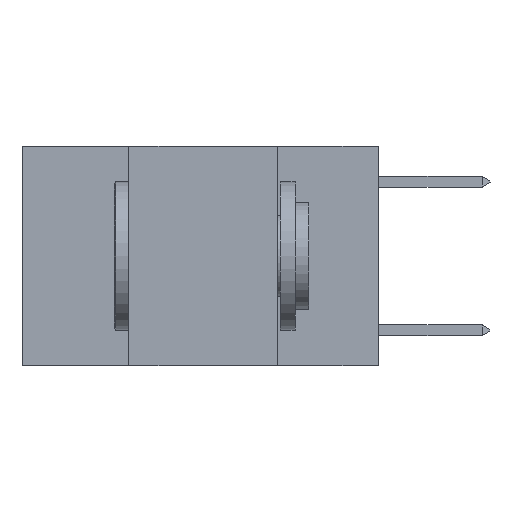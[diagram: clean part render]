
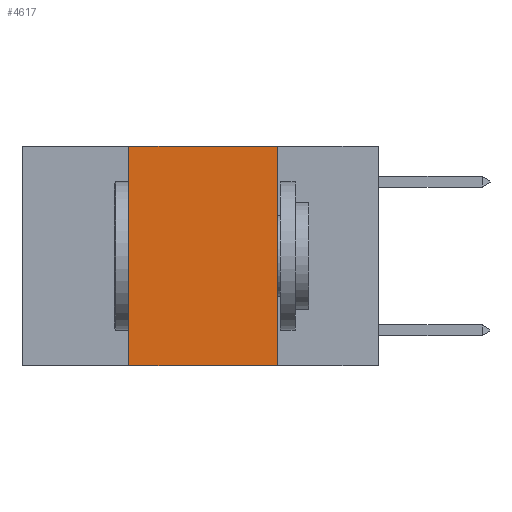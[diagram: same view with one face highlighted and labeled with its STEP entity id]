
A CAD part, left-side view. The second image highlights one B-rep face of the part: STEP entity #4617.
In plain terms, the highlighted planar face has unit normal (-1, 0, 0).
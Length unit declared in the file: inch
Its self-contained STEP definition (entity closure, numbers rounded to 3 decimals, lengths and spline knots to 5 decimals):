
#162 = VERTEX_POINT ( 'NONE', #8802 ) ;
#428 = EDGE_LOOP ( 'NONE', ( #18476, #19750, #6356, #21095 ) ) ;
#827 = VERTEX_POINT ( 'NONE', #20593 ) ;
#1130 = EDGE_CURVE ( 'NONE', #827, #23824, #21213, .T. ) ;
#3015 = DIRECTION ( 'NONE',  ( 0., 0., -1. ) ) ;
#3649 = LINE ( 'NONE', #12258, #13052 ) ;
#3827 = PLANE ( 'NONE',  #18747 ) ;
#4617 = ADVANCED_FACE ( 'NONE', ( #5778 ), #3827, .F. ) ;
#4634 = CARTESIAN_POINT ( 'NONE',  ( 0., 0.42, -0.37 ) ) ;
#5778 = FACE_OUTER_BOUND ( 'NONE', #428, .T. ) ;
#6356 = ORIENTED_EDGE ( 'NONE', *, *, #22737, .F. ) ;
#6431 = VECTOR ( 'NONE', #10769, 39.37008 ) ;
#6537 = DIRECTION ( 'NONE',  ( 0., 0., -1. ) ) ;
#6988 = VECTOR ( 'NONE', #3015, 39.37008 ) ;
#8802 = CARTESIAN_POINT ( 'NONE',  ( 0., 0.17, -0.37 ) ) ;
#9712 = CARTESIAN_POINT ( 'NONE',  ( 0., 0.17, 0. ) ) ;
#10769 = DIRECTION ( 'NONE',  ( 0., -1., 0. ) ) ;
#12258 = CARTESIAN_POINT ( 'NONE',  ( 0., 0.6, -0.37 ) ) ;
#13052 = VECTOR ( 'NONE', #14074, 39.37008 ) ;
#14074 = DIRECTION ( 'NONE',  ( 0., -1., 0. ) ) ;
#14248 = CARTESIAN_POINT ( 'NONE',  ( 0., 0.17, 0. ) ) ;
#15609 = VECTOR ( 'NONE', #19429, 39.37008 ) ;
#17155 = VERTEX_POINT ( 'NONE', #4634 ) ;
#17567 = CARTESIAN_POINT ( 'NONE',  ( 0., 0.42, 0. ) ) ;
#17911 = DIRECTION ( 'NONE',  ( 1., 0., 0. ) ) ;
#18476 = ORIENTED_EDGE ( 'NONE', *, *, #20078, .F. ) ;
#18747 = AXIS2_PLACEMENT_3D ( 'NONE', #21345, #17911, #6537 ) ;
#19429 = DIRECTION ( 'NONE',  ( 0., 0., 1. ) ) ;
#19750 = ORIENTED_EDGE ( 'NONE', *, *, #1130, .F. ) ;
#19925 = LINE ( 'NONE', #17567, #15609 ) ;
#20049 = LINE ( 'NONE', #14248, #6988 ) ;
#20078 = EDGE_CURVE ( 'NONE', #23824, #162, #20049, .T. ) ;
#20593 = CARTESIAN_POINT ( 'NONE',  ( 0., 0.42, 0. ) ) ;
#20804 = CARTESIAN_POINT ( 'NONE',  ( 0., 0.6, 0. ) ) ;
#21095 = ORIENTED_EDGE ( 'NONE', *, *, #23472, .T. ) ;
#21213 = LINE ( 'NONE', #20804, #6431 ) ;
#21345 = CARTESIAN_POINT ( 'NONE',  ( 0., 0.6, 0. ) ) ;
#22737 = EDGE_CURVE ( 'NONE', #17155, #827, #19925, .T. ) ;
#23472 = EDGE_CURVE ( 'NONE', #17155, #162, #3649, .T. ) ;
#23824 = VERTEX_POINT ( 'NONE', #9712 ) ;
